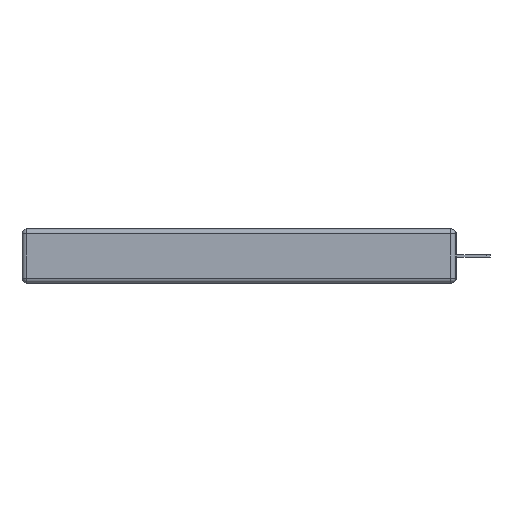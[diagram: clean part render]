
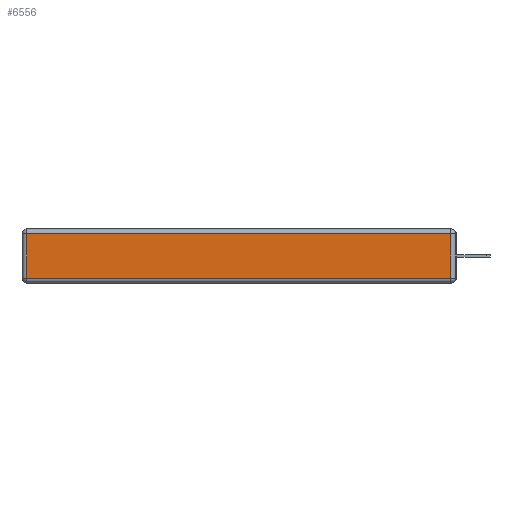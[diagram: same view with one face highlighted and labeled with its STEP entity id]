
A CAD part, left-side view. The second image highlights one B-rep face of the part: STEP entity #6556.
In plain terms, the highlighted planar face has unit normal (-1, 0, 0).
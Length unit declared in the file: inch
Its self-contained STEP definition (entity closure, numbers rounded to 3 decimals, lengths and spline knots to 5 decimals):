
#465 = DIRECTION ( 'NONE',  ( 0., 1., 0. ) ) ;
#1363 = CARTESIAN_POINT ( 'NONE',  ( 0., 2.72, -0.343 ) ) ;
#1433 = AXIS2_PLACEMENT_3D ( 'NONE', #8770, #13575, #3074 ) ;
#2903 = VECTOR ( 'NONE', #465, 39.37008 ) ;
#3074 = DIRECTION ( 'NONE',  ( 0., 0., 1. ) ) ;
#3094 = LINE ( 'NONE', #15312, #10655 ) ;
#3399 = ORIENTED_EDGE ( 'NONE', *, *, #6411, .T. ) ;
#4318 = EDGE_CURVE ( 'NONE', #7759, #7652, #3094, .T. ) ;
#4428 = EDGE_CURVE ( 'NONE', #7652, #9183, #8251, .T. ) ;
#5818 = DIRECTION ( 'NONE',  ( 0., -1., 0. ) ) ;
#5985 = CARTESIAN_POINT ( 'NONE',  ( 0., 2.72, -0.03 ) ) ;
#6411 = EDGE_CURVE ( 'NONE', #7190, #7759, #9554, .T. ) ;
#6556 = ADVANCED_FACE ( 'NONE', ( #7678 ), #6726, .T. ) ;
#6726 = PLANE ( 'NONE',  #1433 ) ;
#6837 = LINE ( 'NONE', #14001, #2903 ) ;
#7190 = VERTEX_POINT ( 'NONE', #5985 ) ;
#7652 = VERTEX_POINT ( 'NONE', #10799 ) ;
#7678 = FACE_OUTER_BOUND ( 'NONE', #9434, .T. ) ;
#7753 = CARTESIAN_POINT ( 'NONE',  ( 0., 2.72, -0.313 ) ) ;
#7759 = VERTEX_POINT ( 'NONE', #7753 ) ;
#8160 = VECTOR ( 'NONE', #13432, 39.37008 ) ;
#8251 = LINE ( 'NONE', #14151, #13378 ) ;
#8770 = CARTESIAN_POINT ( 'NONE',  ( 0., 0., -0.343 ) ) ;
#9183 = VERTEX_POINT ( 'NONE', #11797 ) ;
#9209 = ORIENTED_EDGE ( 'NONE', *, *, #12511, .T. ) ;
#9434 = EDGE_LOOP ( 'NONE', ( #13683, #10937, #9209, #3399 ) ) ;
#9554 = LINE ( 'NONE', #1363, #8160 ) ;
#10647 = DIRECTION ( 'NONE',  ( 0., 0., 1. ) ) ;
#10655 = VECTOR ( 'NONE', #5818, 39.37008 ) ;
#10799 = CARTESIAN_POINT ( 'NONE',  ( 0., 0.03, -0.313 ) ) ;
#10937 = ORIENTED_EDGE ( 'NONE', *, *, #4428, .T. ) ;
#11797 = CARTESIAN_POINT ( 'NONE',  ( 0., 0.03, -0.03 ) ) ;
#12511 = EDGE_CURVE ( 'NONE', #9183, #7190, #6837, .T. ) ;
#13378 = VECTOR ( 'NONE', #10647, 39.37008 ) ;
#13432 = DIRECTION ( 'NONE',  ( 0., 0., -1. ) ) ;
#13575 = DIRECTION ( 'NONE',  ( -1., 0., 0. ) ) ;
#13683 = ORIENTED_EDGE ( 'NONE', *, *, #4318, .T. ) ;
#14001 = CARTESIAN_POINT ( 'NONE',  ( 0., 2.75, -0.03 ) ) ;
#14151 = CARTESIAN_POINT ( 'NONE',  ( 0., 0.03, -0.343 ) ) ;
#15312 = CARTESIAN_POINT ( 'NONE',  ( 0., 0., -0.313 ) ) ;
